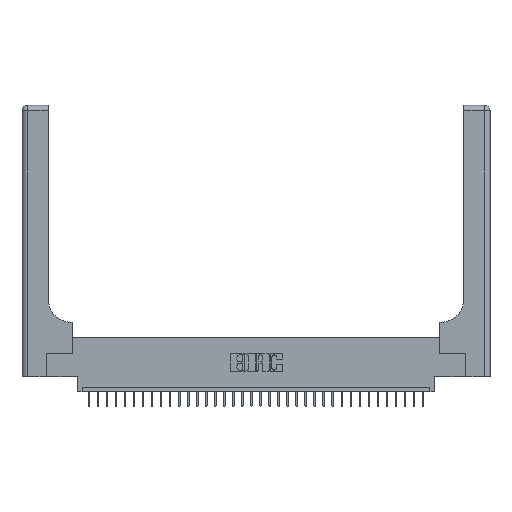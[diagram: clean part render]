
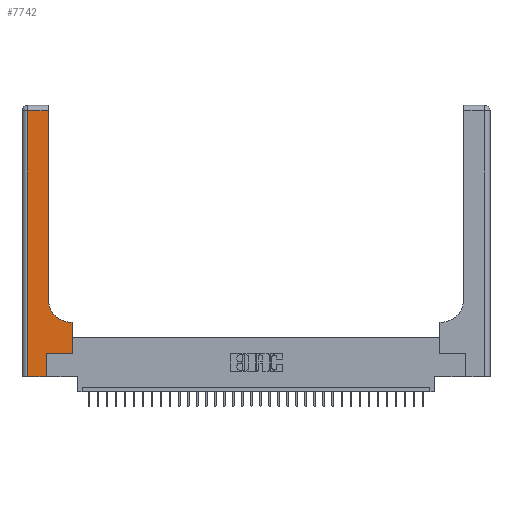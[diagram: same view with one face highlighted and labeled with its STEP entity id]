
A CAD part, top view. The second image highlights one B-rep face of the part: STEP entity #7742.
In plain terms, the highlighted planar face has unit normal (0, 0, 1).
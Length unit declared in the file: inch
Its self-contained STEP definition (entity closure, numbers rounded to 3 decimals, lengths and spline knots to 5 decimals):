
#97 = ORIENTED_EDGE ( 'NONE', *, *, #13523, .T. ) ;
#541 = VERTEX_POINT ( 'NONE', #7525 ) ;
#731 = LINE ( 'NONE', #22673, #30773 ) ;
#1016 = EDGE_CURVE ( 'NONE', #7273, #1628, #27864, .T. ) ;
#1147 = LINE ( 'NONE', #13603, #28644 ) ;
#1470 = DIRECTION ( 'NONE',  ( 0., 1., 0. ) ) ;
#1628 = VERTEX_POINT ( 'NONE', #18327 ) ;
#1852 = CARTESIAN_POINT ( 'NONE',  ( 0.2915, 0.85, 0.37 ) ) ;
#2381 = CARTESIAN_POINT ( 'NONE',  ( 0.5415, 0.85, 0.37 ) ) ;
#2540 = LINE ( 'NONE', #26011, #11685 ) ;
#4107 = VECTOR ( 'NONE', #24343, 39.37008 ) ;
#6665 = CIRCLE ( 'NONE', #24530, 0.25 ) ;
#7111 = ORIENTED_EDGE ( 'NONE', *, *, #18390, .T. ) ;
#7273 = VERTEX_POINT ( 'NONE', #18853 ) ;
#7525 = CARTESIAN_POINT ( 'NONE',  ( 0.269, 0.25, 0.37 ) ) ;
#7536 = CARTESIAN_POINT ( 'NONE',  ( 0.269, 0., 0.37 ) ) ;
#7742 = ADVANCED_FACE ( 'NONE', ( #16930 ), #26698, .F. ) ;
#8283 = CARTESIAN_POINT ( 'NONE',  ( 0., 3., 0.37 ) ) ;
#8897 = AXIS2_PLACEMENT_3D ( 'NONE', #8283, #16420, #13627 ) ;
#9413 = DIRECTION ( 'NONE',  ( -1., 0., 0. ) ) ;
#9490 = VERTEX_POINT ( 'NONE', #19906 ) ;
#11178 = EDGE_CURVE ( 'NONE', #1628, #541, #31717, .T. ) ;
#11673 = CARTESIAN_POINT ( 'NONE',  ( 0.5415, 0.6, 0.37 ) ) ;
#11685 = VECTOR ( 'NONE', #28658, 39.37008 ) ;
#11717 = EDGE_CURVE ( 'NONE', #33922, #7273, #2540, .T. ) ;
#12732 = CARTESIAN_POINT ( 'NONE',  ( 0.269, 0.25, 0.37 ) ) ;
#12904 = VECTOR ( 'NONE', #24722, 39.37008 ) ;
#13523 = EDGE_CURVE ( 'NONE', #9490, #29883, #1147, .T. ) ;
#13603 = CARTESIAN_POINT ( 'NONE',  ( 0.2915, 0.6, 0.37 ) ) ;
#13627 = DIRECTION ( 'NONE',  ( -1., 0., 0. ) ) ;
#13758 = EDGE_CURVE ( 'NONE', #16415, #9490, #731, .T. ) ;
#13775 = DIRECTION ( 'NONE',  ( 0., 1., 0. ) ) ;
#14731 = EDGE_CURVE ( 'NONE', #24619, #22855, #19769, .T. ) ;
#15182 = LINE ( 'NONE', #22474, #24831 ) ;
#16151 = ORIENTED_EDGE ( 'NONE', *, *, #11178, .T. ) ;
#16191 = ORIENTED_EDGE ( 'NONE', *, *, #1016, .T. ) ;
#16415 = VERTEX_POINT ( 'NONE', #25588 ) ;
#16420 = DIRECTION ( 'NONE',  ( 0., 0., -1. ) ) ;
#16930 = FACE_OUTER_BOUND ( 'NONE', #19762, .T. ) ;
#18327 = CARTESIAN_POINT ( 'NONE',  ( 0.269, 0., 0.37 ) ) ;
#18390 = EDGE_CURVE ( 'NONE', #29883, #24619, #6665, .T. ) ;
#18852 = LINE ( 'NONE', #12732, #34390 ) ;
#18853 = CARTESIAN_POINT ( 'NONE',  ( 0.06, 0., 0.37 ) ) ;
#19762 = EDGE_LOOP ( 'NONE', ( #32682, #32507, #34042, #16191, #16151, #26756, #32537, #97, #7111 ) ) ;
#19769 = LINE ( 'NONE', #29761, #31495 ) ;
#19906 = CARTESIAN_POINT ( 'NONE',  ( 0.5585, 0.6, 0.37 ) ) ;
#20994 = DIRECTION ( 'NONE',  ( 1., 0., 0. ) ) ;
#21704 = EDGE_CURVE ( 'NONE', #541, #16415, #18852, .T. ) ;
#21901 = DIRECTION ( 'NONE',  ( -1., 0., 0. ) ) ;
#22474 = CARTESIAN_POINT ( 'NONE',  ( 0., 2.94, 0.37 ) ) ;
#22673 = CARTESIAN_POINT ( 'NONE',  ( 0.5585, 0.25, 0.37 ) ) ;
#22855 = VERTEX_POINT ( 'NONE', #27872 ) ;
#24343 = DIRECTION ( 'NONE',  ( 1., 0., 0. ) ) ;
#24530 = AXIS2_PLACEMENT_3D ( 'NONE', #2381, #31281, #20994 ) ;
#24619 = VERTEX_POINT ( 'NONE', #1852 ) ;
#24683 = CARTESIAN_POINT ( 'NONE',  ( 0.06, 2.94, 0.37 ) ) ;
#24722 = DIRECTION ( 'NONE',  ( 0., 1., 0. ) ) ;
#24831 = VECTOR ( 'NONE', #9413, 39.37008 ) ;
#25548 = EDGE_CURVE ( 'NONE', #22855, #33922, #15182, .T. ) ;
#25588 = CARTESIAN_POINT ( 'NONE',  ( 0.5585, 0.25, 0.37 ) ) ;
#26011 = CARTESIAN_POINT ( 'NONE',  ( 0.06, 3., 0.37 ) ) ;
#26277 = DIRECTION ( 'NONE',  ( 1., 0., 0. ) ) ;
#26698 = PLANE ( 'NONE',  #8897 ) ;
#26756 = ORIENTED_EDGE ( 'NONE', *, *, #21704, .T. ) ;
#27237 = CARTESIAN_POINT ( 'NONE',  ( 0., 0., 0.37 ) ) ;
#27864 = LINE ( 'NONE', #27237, #4107 ) ;
#27872 = CARTESIAN_POINT ( 'NONE',  ( 0.2915, 2.94, 0.37 ) ) ;
#28644 = VECTOR ( 'NONE', #21901, 39.37008 ) ;
#28658 = DIRECTION ( 'NONE',  ( 0., -1., 0. ) ) ;
#29761 = CARTESIAN_POINT ( 'NONE',  ( 0.2915, 3., 0.37 ) ) ;
#29883 = VERTEX_POINT ( 'NONE', #11673 ) ;
#30773 = VECTOR ( 'NONE', #1470, 39.37008 ) ;
#31281 = DIRECTION ( 'NONE',  ( 0., 0., -1. ) ) ;
#31495 = VECTOR ( 'NONE', #13775, 39.37008 ) ;
#31717 = LINE ( 'NONE', #7536, #12904 ) ;
#32507 = ORIENTED_EDGE ( 'NONE', *, *, #25548, .T. ) ;
#32537 = ORIENTED_EDGE ( 'NONE', *, *, #13758, .T. ) ;
#32682 = ORIENTED_EDGE ( 'NONE', *, *, #14731, .T. ) ;
#33922 = VERTEX_POINT ( 'NONE', #24683 ) ;
#34042 = ORIENTED_EDGE ( 'NONE', *, *, #11717, .T. ) ;
#34390 = VECTOR ( 'NONE', #26277, 39.37008 ) ;
